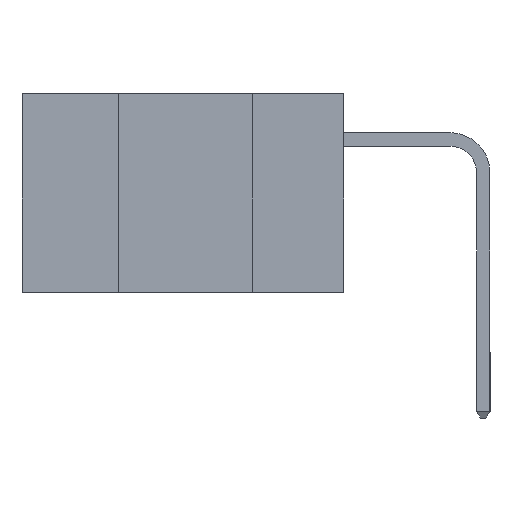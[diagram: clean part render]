
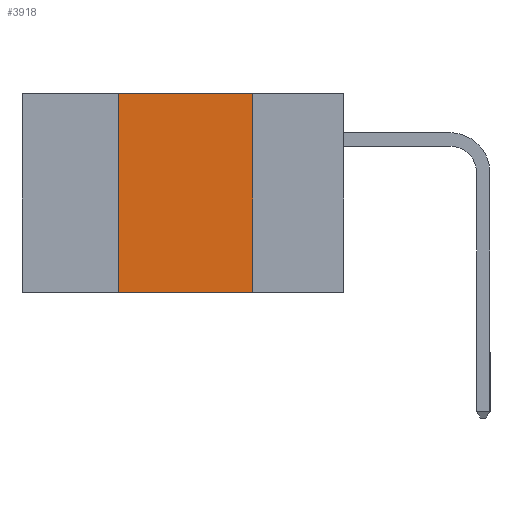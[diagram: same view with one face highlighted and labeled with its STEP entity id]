
A CAD part, left-side view. The second image highlights one B-rep face of the part: STEP entity #3918.
In plain terms, the highlighted planar face has unit normal (-1, 0, 0).
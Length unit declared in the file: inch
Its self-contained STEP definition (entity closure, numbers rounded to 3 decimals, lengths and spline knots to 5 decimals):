
#285 = DIRECTION ( 'NONE',  ( 0., -1., 0. ) ) ;
#1067 = CARTESIAN_POINT ( 'NONE',  ( 0., 0.17, 0. ) ) ;
#1493 = LINE ( 'NONE', #1613, #8561 ) ;
#1613 = CARTESIAN_POINT ( 'NONE',  ( 0., 0.6, 0. ) ) ;
#1653 = VERTEX_POINT ( 'NONE', #1067 ) ;
#2461 = ORIENTED_EDGE ( 'NONE', *, *, #7504, .F. ) ;
#2500 = VERTEX_POINT ( 'NONE', #6065 ) ;
#2744 = VECTOR ( 'NONE', #3747, 39.37008 ) ;
#3747 = DIRECTION ( 'NONE',  ( 0., -1., 0. ) ) ;
#3822 = CARTESIAN_POINT ( 'NONE',  ( 0., 0.42, -0.37 ) ) ;
#3918 = ADVANCED_FACE ( 'NONE', ( #8920 ), #12469, .F. ) ;
#4069 = VERTEX_POINT ( 'NONE', #12174 ) ;
#4214 = CARTESIAN_POINT ( 'NONE',  ( 0., 0.42, 0. ) ) ;
#4632 = LINE ( 'NONE', #10845, #2744 ) ;
#5549 = LINE ( 'NONE', #6044, #6465 ) ;
#5576 = ORIENTED_EDGE ( 'NONE', *, *, #13345, .F. ) ;
#6044 = CARTESIAN_POINT ( 'NONE',  ( 0., 0.17, 0. ) ) ;
#6065 = CARTESIAN_POINT ( 'NONE',  ( 0., 0.42, 0. ) ) ;
#6287 = VECTOR ( 'NONE', #7773, 39.37008 ) ;
#6465 = VECTOR ( 'NONE', #15418, 39.37008 ) ;
#6482 = LINE ( 'NONE', #4214, #6287 ) ;
#6542 = DIRECTION ( 'NONE',  ( 0., 0., -1. ) ) ;
#7324 = EDGE_CURVE ( 'NONE', #15336, #4069, #4632, .T. ) ;
#7504 = EDGE_CURVE ( 'NONE', #1653, #4069, #5549, .T. ) ;
#7773 = DIRECTION ( 'NONE',  ( 0., 0., 1. ) ) ;
#8561 = VECTOR ( 'NONE', #285, 39.37008 ) ;
#8920 = FACE_OUTER_BOUND ( 'NONE', #9999, .T. ) ;
#9264 = ORIENTED_EDGE ( 'NONE', *, *, #7324, .T. ) ;
#9999 = EDGE_LOOP ( 'NONE', ( #2461, #5576, #10690, #9264 ) ) ;
#10690 = ORIENTED_EDGE ( 'NONE', *, *, #10698, .F. ) ;
#10698 = EDGE_CURVE ( 'NONE', #15336, #2500, #6482, .T. ) ;
#10845 = CARTESIAN_POINT ( 'NONE',  ( 0., 0.6, -0.37 ) ) ;
#12174 = CARTESIAN_POINT ( 'NONE',  ( 0., 0.17, -0.37 ) ) ;
#12336 = AXIS2_PLACEMENT_3D ( 'NONE', #13651, #13704, #6542 ) ;
#12469 = PLANE ( 'NONE',  #12336 ) ;
#13345 = EDGE_CURVE ( 'NONE', #2500, #1653, #1493, .T. ) ;
#13651 = CARTESIAN_POINT ( 'NONE',  ( 0., 0.6, 0. ) ) ;
#13704 = DIRECTION ( 'NONE',  ( 1., 0., 0. ) ) ;
#15336 = VERTEX_POINT ( 'NONE', #3822 ) ;
#15418 = DIRECTION ( 'NONE',  ( 0., 0., -1. ) ) ;
